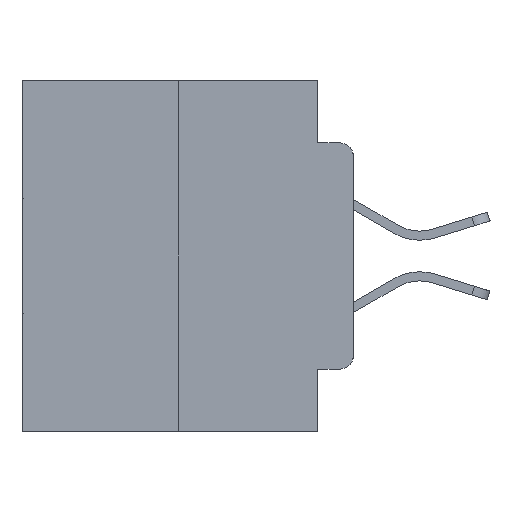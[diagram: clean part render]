
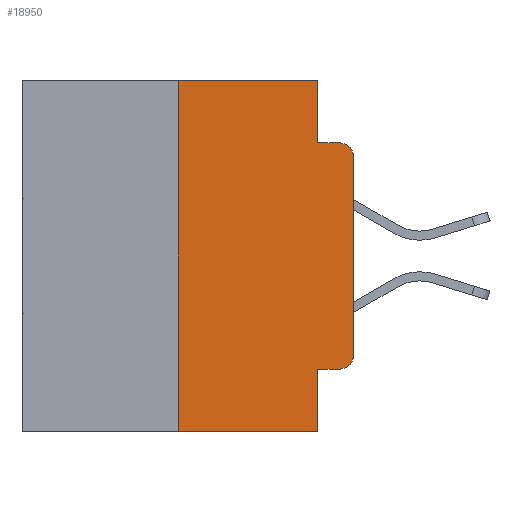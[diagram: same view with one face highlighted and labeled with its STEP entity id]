
A CAD part, left-side view. The second image highlights one B-rep face of the part: STEP entity #18950.
In plain terms, the highlighted planar face has unit normal (-1, 0, 0).
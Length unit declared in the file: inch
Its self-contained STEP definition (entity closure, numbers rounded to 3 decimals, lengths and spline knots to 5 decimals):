
#200 = AXIS2_PLACEMENT_3D ( 'NONE', #11900, #20627, #24968 ) ;
#225 = CIRCLE ( 'NONE', #22497, 0.02 ) ;
#1201 = VERTEX_POINT ( 'NONE', #8515 ) ;
#1860 = VECTOR ( 'NONE', #27589, 39.37008 ) ;
#1989 = CARTESIAN_POINT ( 'NONE',  ( 0., 0.25, 0. ) ) ;
#2179 = LINE ( 'NONE', #13106, #18956 ) ;
#2315 = EDGE_CURVE ( 'NONE', #26808, #18919, #2578, .T. ) ;
#2578 = LINE ( 'NONE', #1989, #10527 ) ;
#2752 = CARTESIAN_POINT ( 'NONE',  ( 0., 0.25, 0. ) ) ;
#2875 = CARTESIAN_POINT ( 'NONE',  ( 0., 0.051, -0.5 ) ) ;
#4257 = CARTESIAN_POINT ( 'NONE',  ( 0., 0., 0. ) ) ;
#4699 = VECTOR ( 'NONE', #21653, 39.37008 ) ;
#5218 = CARTESIAN_POINT ( 'NONE',  ( 0., 0.02, -0.3915 ) ) ;
#5608 = CARTESIAN_POINT ( 'NONE',  ( 0., 0.02, -0.1085 ) ) ;
#5824 = VECTOR ( 'NONE', #19090, 39.37008 ) ;
#5892 = AXIS2_PLACEMENT_3D ( 'NONE', #5608, #25213, #27532 ) ;
#6100 = ORIENTED_EDGE ( 'NONE', *, *, #2315, .F. ) ;
#7360 = ORIENTED_EDGE ( 'NONE', *, *, #11286, .T. ) ;
#7601 = CARTESIAN_POINT ( 'NONE',  ( 0., 0.051, 0. ) ) ;
#8256 = VERTEX_POINT ( 'NONE', #18937 ) ;
#8515 = CARTESIAN_POINT ( 'NONE',  ( 0., 0.02, -0.4115 ) ) ;
#8610 = LINE ( 'NONE', #4257, #26952 ) ;
#8655 = EDGE_LOOP ( 'NONE', ( #7360, #19149, #16703, #10681, #26749, #6100, #26476, #24442, #14487, #9306 ) ) ;
#9306 = ORIENTED_EDGE ( 'NONE', *, *, #19033, .T. ) ;
#9728 = DIRECTION ( 'NONE',  ( 0., -1., 0. ) ) ;
#9846 = DIRECTION ( 'NONE',  ( -1., 0., 0. ) ) ;
#9850 = CARTESIAN_POINT ( 'NONE',  ( 0., 0.051, -0.4115 ) ) ;
#10527 = VECTOR ( 'NONE', #13348, 39.37008 ) ;
#10681 = ORIENTED_EDGE ( 'NONE', *, *, #27514, .F. ) ;
#10715 = LINE ( 'NONE', #15389, #4699 ) ;
#10900 = DIRECTION ( 'NONE',  ( 0., -1., 0. ) ) ;
#11286 = EDGE_CURVE ( 'NONE', #22903, #12567, #8610, .T. ) ;
#11440 = CIRCLE ( 'NONE', #5892, 0.02 ) ;
#11607 = FACE_OUTER_BOUND ( 'NONE', #8655, .T. ) ;
#11726 = EDGE_CURVE ( 'NONE', #18919, #16076, #2179, .T. ) ;
#11900 = CARTESIAN_POINT ( 'NONE',  ( 0., 0.473, 0. ) ) ;
#12567 = VERTEX_POINT ( 'NONE', #12724 ) ;
#12724 = CARTESIAN_POINT ( 'NONE',  ( 0., 0., -0.1085 ) ) ;
#13106 = CARTESIAN_POINT ( 'NONE',  ( 0., 0.473, 0. ) ) ;
#13348 = DIRECTION ( 'NONE',  ( 0., 0., 1. ) ) ;
#13781 = VERTEX_POINT ( 'NONE', #2875 ) ;
#13952 = CARTESIAN_POINT ( 'NONE',  ( 0., 0.051, 0. ) ) ;
#14121 = LINE ( 'NONE', #9850, #1860 ) ;
#14487 = ORIENTED_EDGE ( 'NONE', *, *, #27052, .T. ) ;
#15389 = CARTESIAN_POINT ( 'NONE',  ( 0., 0.051, 0. ) ) ;
#16076 = VERTEX_POINT ( 'NONE', #13952 ) ;
#16703 = ORIENTED_EDGE ( 'NONE', *, *, #17048, .F. ) ;
#17048 = EDGE_CURVE ( 'NONE', #25727, #22506, #21982, .T. ) ;
#17345 = EDGE_CURVE ( 'NONE', #26808, #13781, #18785, .T. ) ;
#18186 = CARTESIAN_POINT ( 'NONE',  ( 0., 0.051, -0.0885 ) ) ;
#18785 = LINE ( 'NONE', #20511, #28421 ) ;
#18919 = VERTEX_POINT ( 'NONE', #2752 ) ;
#18937 = CARTESIAN_POINT ( 'NONE',  ( 0., 0.051, -0.4115 ) ) ;
#18950 = ADVANCED_FACE ( 'NONE', ( #11607 ), #27585, .F. ) ;
#18956 = VECTOR ( 'NONE', #10900, 39.37008 ) ;
#19033 = EDGE_CURVE ( 'NONE', #1201, #22903, #225, .T. ) ;
#19090 = DIRECTION ( 'NONE',  ( 0., 0., -1. ) ) ;
#19149 = ORIENTED_EDGE ( 'NONE', *, *, #22770, .T. ) ;
#20511 = CARTESIAN_POINT ( 'NONE',  ( 0., 0.473, -0.5 ) ) ;
#20627 = DIRECTION ( 'NONE',  ( 1., 0., 0. ) ) ;
#21055 = DIRECTION ( 'NONE',  ( 0., 0., -1. ) ) ;
#21538 = EDGE_CURVE ( 'NONE', #8256, #13781, #27487, .T. ) ;
#21653 = DIRECTION ( 'NONE',  ( 0., 0., -1. ) ) ;
#21982 = LINE ( 'NONE', #24126, #25607 ) ;
#22497 = AXIS2_PLACEMENT_3D ( 'NONE', #5218, #9846, #21055 ) ;
#22506 = VERTEX_POINT ( 'NONE', #28585 ) ;
#22770 = EDGE_CURVE ( 'NONE', #12567, #22506, #11440, .T. ) ;
#22903 = VERTEX_POINT ( 'NONE', #24024 ) ;
#24024 = CARTESIAN_POINT ( 'NONE',  ( 0., 0., -0.3915 ) ) ;
#24126 = CARTESIAN_POINT ( 'NONE',  ( 0., 0.051, -0.0885 ) ) ;
#24442 = ORIENTED_EDGE ( 'NONE', *, *, #21538, .F. ) ;
#24968 = DIRECTION ( 'NONE',  ( 0., 0., -1. ) ) ;
#25213 = DIRECTION ( 'NONE',  ( -1., 0., 0. ) ) ;
#25607 = VECTOR ( 'NONE', #28224, 39.37008 ) ;
#25727 = VERTEX_POINT ( 'NONE', #18186 ) ;
#26476 = ORIENTED_EDGE ( 'NONE', *, *, #17345, .T. ) ;
#26749 = ORIENTED_EDGE ( 'NONE', *, *, #11726, .F. ) ;
#26808 = VERTEX_POINT ( 'NONE', #27001 ) ;
#26952 = VECTOR ( 'NONE', #28236, 39.37008 ) ;
#27001 = CARTESIAN_POINT ( 'NONE',  ( 0., 0.25, -0.5 ) ) ;
#27052 = EDGE_CURVE ( 'NONE', #8256, #1201, #14121, .T. ) ;
#27487 = LINE ( 'NONE', #7601, #5824 ) ;
#27514 = EDGE_CURVE ( 'NONE', #16076, #25727, #10715, .T. ) ;
#27532 = DIRECTION ( 'NONE',  ( 0., 0., -1. ) ) ;
#27585 = PLANE ( 'NONE',  #200 ) ;
#27589 = DIRECTION ( 'NONE',  ( 0., -1., 0. ) ) ;
#28224 = DIRECTION ( 'NONE',  ( 0., -1., 0. ) ) ;
#28236 = DIRECTION ( 'NONE',  ( 0., 0., 1. ) ) ;
#28421 = VECTOR ( 'NONE', #9728, 39.37008 ) ;
#28585 = CARTESIAN_POINT ( 'NONE',  ( 0., 0.02, -0.0885 ) ) ;
